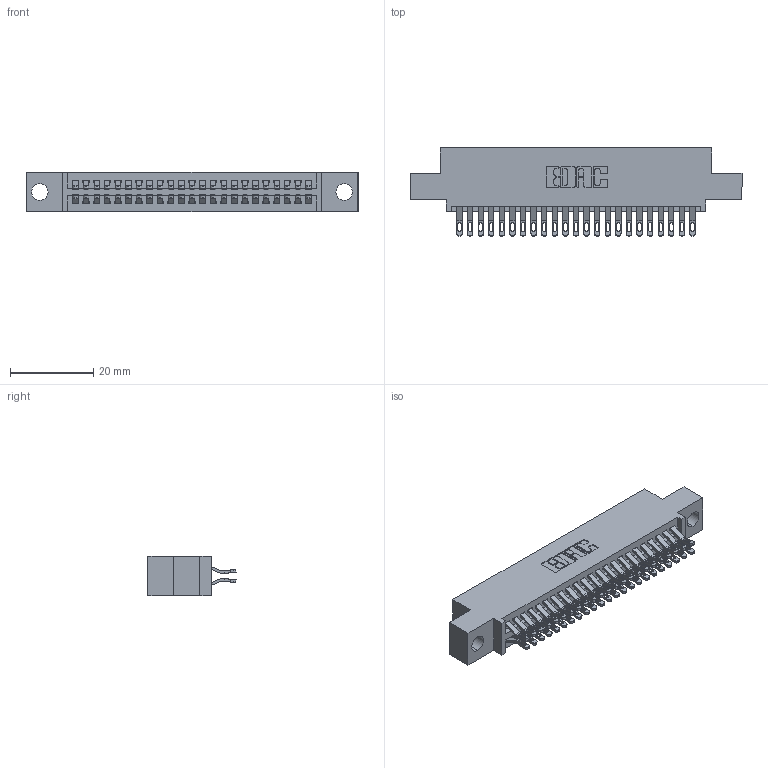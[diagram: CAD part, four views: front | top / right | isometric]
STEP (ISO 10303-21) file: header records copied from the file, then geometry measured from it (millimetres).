
FILE_DESCRIPTION (( 'STEP AP203' ), '1' );
FILE_NAME ('345-046-555-504.STEP', '2021-05-20T02:28:45', ( '' ), ( '' ), 'SwSTEP 2.0', 'SolidWorks 2020', '' );
FILE_SCHEMA (( 'CONFIG_CONTROL_DESIGN' ));
Length unit declared in the file: inch
Products named in the file (3): 345-046-555-504; 345 Part_0.110 Offset - 0.156 Dia-TI; 345-292-001_555 Tail
Assembly tree (47 placements, depth 2):
  345-046-555-504
    345 Part_0.110 Offset - 0.156 Dia-TI
    345-292-001_555 Tail  x46
Bounding box: 79.63 x 21.13 x 9.4 mm (x, y, z)
Volume: 7513 mm3; surface area: 11146 mm2
Topology: 47 solids, 47 shells, 2720 faces, 8531 edges, 5686 vertices
Faces by surface type: plane 1524, cylinder 1196
Entity records: 21481 total; most frequent: CARTESIAN_POINT 3660, ORIENTED_EDGE 3562, DIRECTION 3217, EDGE_CURVE 1781, VECTOR 1537, LINE 1537, VERTEX_POINT 1186, AXIS2_PLACEMENT_3D 840
